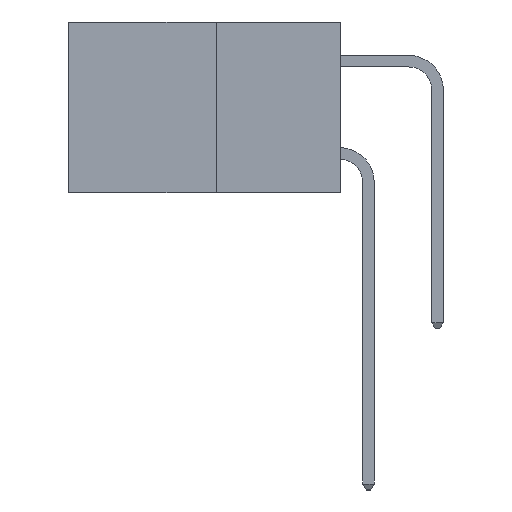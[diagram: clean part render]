
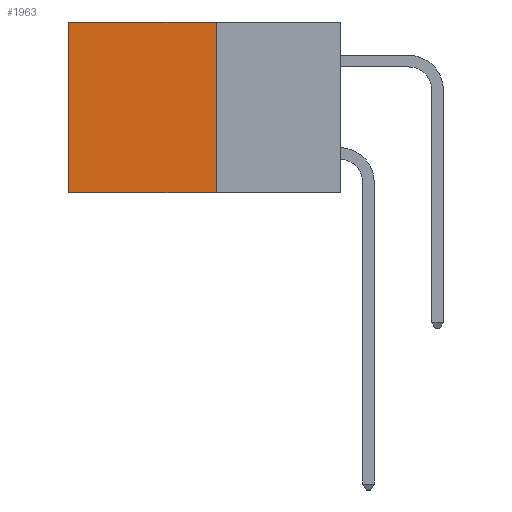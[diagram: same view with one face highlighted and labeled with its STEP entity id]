
A CAD part, left-side view. The second image highlights one B-rep face of the part: STEP entity #1963.
In plain terms, the highlighted planar face has unit normal (-1, 0, 0).
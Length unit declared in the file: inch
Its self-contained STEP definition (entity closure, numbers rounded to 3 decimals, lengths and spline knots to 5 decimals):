
#120 = ORIENTED_EDGE ( 'NONE', *, *, #3247, .T. ) ;
#228 = CARTESIAN_POINT ( 'NONE',  ( 0.277, 0.27, 0. ) ) ;
#657 = VECTOR ( 'NONE', #9314, 39.37008 ) ;
#1798 = CARTESIAN_POINT ( 'NONE',  ( 0.277, 0.27, -0.37 ) ) ;
#1864 = DIRECTION ( 'NONE',  ( 0., 1., 0. ) ) ;
#1963 = ADVANCED_FACE ( 'NONE', ( #9934 ), #3661, .F. ) ;
#2686 = EDGE_CURVE ( 'NONE', #11942, #13676, #3526, .T. ) ;
#2997 = DIRECTION ( 'NONE',  ( 0., 1., 0. ) ) ;
#3247 = EDGE_CURVE ( 'NONE', #8461, #5339, #10822, .T. ) ;
#3526 = LINE ( 'NONE', #8864, #6568 ) ;
#3555 = EDGE_CURVE ( 'NONE', #5339, #13676, #3845, .T. ) ;
#3636 = VECTOR ( 'NONE', #7097, 39.37008 ) ;
#3661 = PLANE ( 'NONE',  #10196 ) ;
#3845 = LINE ( 'NONE', #9529, #657 ) ;
#4307 = EDGE_LOOP ( 'NONE', ( #11795, #4857, #10848, #120 ) ) ;
#4708 = EDGE_CURVE ( 'NONE', #8461, #11942, #9698, .T. ) ;
#4857 = ORIENTED_EDGE ( 'NONE', *, *, #2686, .F. ) ;
#5339 = VERTEX_POINT ( 'NONE', #13864 ) ;
#5860 = CARTESIAN_POINT ( 'NONE',  ( 0.277, 0.27, -0.37 ) ) ;
#6129 = DIRECTION ( 'NONE',  ( 1., 0., 0. ) ) ;
#6568 = VECTOR ( 'NONE', #2997, 39.37008 ) ;
#6842 = CARTESIAN_POINT ( 'NONE',  ( 0.277, 0.27, -0.37 ) ) ;
#6997 = CARTESIAN_POINT ( 'NONE',  ( 0.277, 0.59, -0.37 ) ) ;
#7097 = DIRECTION ( 'NONE',  ( 0., 0., -1. ) ) ;
#8461 = VERTEX_POINT ( 'NONE', #228 ) ;
#8864 = CARTESIAN_POINT ( 'NONE',  ( 0.277, 0.27, -0.37 ) ) ;
#9314 = DIRECTION ( 'NONE',  ( 0., 0., -1. ) ) ;
#9529 = CARTESIAN_POINT ( 'NONE',  ( 0.277, 0.59, -0.37 ) ) ;
#9698 = LINE ( 'NONE', #6842, #3636 ) ;
#9934 = FACE_OUTER_BOUND ( 'NONE', #4307, .T. ) ;
#10196 = AXIS2_PLACEMENT_3D ( 'NONE', #5860, #6129, #10497 ) ;
#10497 = DIRECTION ( 'NONE',  ( 0., 0., -1. ) ) ;
#10822 = LINE ( 'NONE', #14305, #11188 ) ;
#10848 = ORIENTED_EDGE ( 'NONE', *, *, #4708, .F. ) ;
#11188 = VECTOR ( 'NONE', #1864, 39.37008 ) ;
#11795 = ORIENTED_EDGE ( 'NONE', *, *, #3555, .T. ) ;
#11942 = VERTEX_POINT ( 'NONE', #1798 ) ;
#13676 = VERTEX_POINT ( 'NONE', #6997 ) ;
#13864 = CARTESIAN_POINT ( 'NONE',  ( 0.277, 0.59, 0. ) ) ;
#14305 = CARTESIAN_POINT ( 'NONE',  ( 0.277, 0.27, 0. ) ) ;
